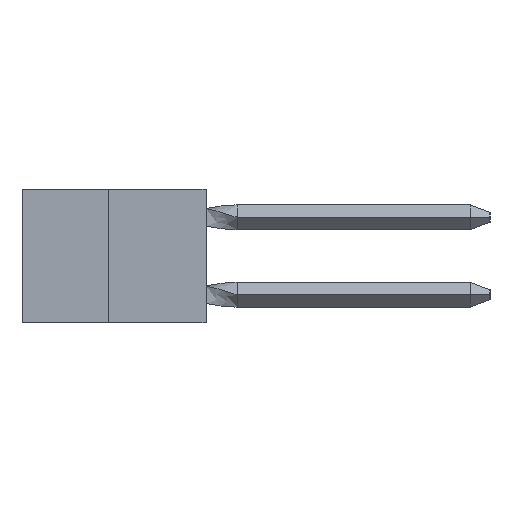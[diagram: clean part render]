
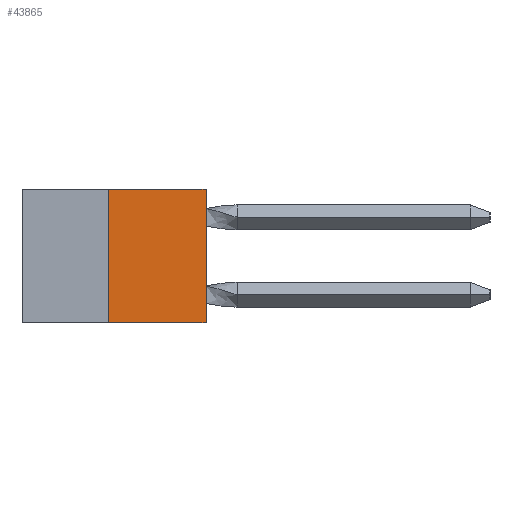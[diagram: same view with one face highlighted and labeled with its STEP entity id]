
A CAD part, left-side view. The second image highlights one B-rep face of the part: STEP entity #43865.
In plain terms, the highlighted planar face has unit normal (-1, 0, 0).
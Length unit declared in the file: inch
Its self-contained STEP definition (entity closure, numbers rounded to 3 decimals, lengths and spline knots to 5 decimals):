
#2123 = PLANE ( 'NONE',  #46064 ) ;
#4324 = VECTOR ( 'NONE', #9063, 39.37008 ) ;
#4533 = CARTESIAN_POINT ( 'NONE',  ( 0., 0.25, -0.343 ) ) ;
#5645 = VERTEX_POINT ( 'NONE', #4533 ) ;
#6909 = EDGE_CURVE ( 'NONE', #5645, #27955, #47994, .T. ) ;
#7542 = EDGE_LOOP ( 'NONE', ( #33242, #39699, #12964, #33713 ) ) ;
#9063 = DIRECTION ( 'NONE',  ( 0., 0., 1. ) ) ;
#10664 = DIRECTION ( 'NONE',  ( 0., -1., 0. ) ) ;
#12964 = ORIENTED_EDGE ( 'NONE', *, *, #23187, .T. ) ;
#16098 = CARTESIAN_POINT ( 'NONE',  ( 0., 0.25, 0. ) ) ;
#16986 = CARTESIAN_POINT ( 'NONE',  ( 0., 0., 0. ) ) ;
#18021 = CARTESIAN_POINT ( 'NONE',  ( 0., 0.473, 0. ) ) ;
#18771 = LINE ( 'NONE', #40644, #56718 ) ;
#19383 = CARTESIAN_POINT ( 'NONE',  ( 0., 0.25, 0. ) ) ;
#20994 = EDGE_CURVE ( 'NONE', #40816, #43316, #33209, .T. ) ;
#21881 = VECTOR ( 'NONE', #23617, 39.37008 ) ;
#23187 = EDGE_CURVE ( 'NONE', #5645, #40816, #18771, .T. ) ;
#23617 = DIRECTION ( 'NONE',  ( 0., 0., 1. ) ) ;
#27389 = CARTESIAN_POINT ( 'NONE',  ( 0., 0., 0. ) ) ;
#27955 = VERTEX_POINT ( 'NONE', #16098 ) ;
#28277 = DIRECTION ( 'NONE',  ( 0., 0., -1. ) ) ;
#33209 = LINE ( 'NONE', #16986, #4324 ) ;
#33242 = ORIENTED_EDGE ( 'NONE', *, *, #43248, .F. ) ;
#33713 = ORIENTED_EDGE ( 'NONE', *, *, #20994, .T. ) ;
#36285 = LINE ( 'NONE', #18021, #38345 ) ;
#38345 = VECTOR ( 'NONE', #10664, 39.37008 ) ;
#39699 = ORIENTED_EDGE ( 'NONE', *, *, #6909, .F. ) ;
#40093 = DIRECTION ( 'NONE',  ( 0., -1., 0. ) ) ;
#40644 = CARTESIAN_POINT ( 'NONE',  ( 0., 0.473, -0.343 ) ) ;
#40816 = VERTEX_POINT ( 'NONE', #41632 ) ;
#41632 = CARTESIAN_POINT ( 'NONE',  ( 0., 0., -0.343 ) ) ;
#43248 = EDGE_CURVE ( 'NONE', #27955, #43316, #36285, .T. ) ;
#43316 = VERTEX_POINT ( 'NONE', #27389 ) ;
#43865 = ADVANCED_FACE ( 'NONE', ( #47210 ), #2123, .F. ) ;
#45743 = DIRECTION ( 'NONE',  ( 1., 0., 0. ) ) ;
#46064 = AXIS2_PLACEMENT_3D ( 'NONE', #49633, #45743, #28277 ) ;
#47210 = FACE_OUTER_BOUND ( 'NONE', #7542, .T. ) ;
#47994 = LINE ( 'NONE', #19383, #21881 ) ;
#49633 = CARTESIAN_POINT ( 'NONE',  ( 0., 0.473, 0. ) ) ;
#56718 = VECTOR ( 'NONE', #40093, 39.37008 ) ;
